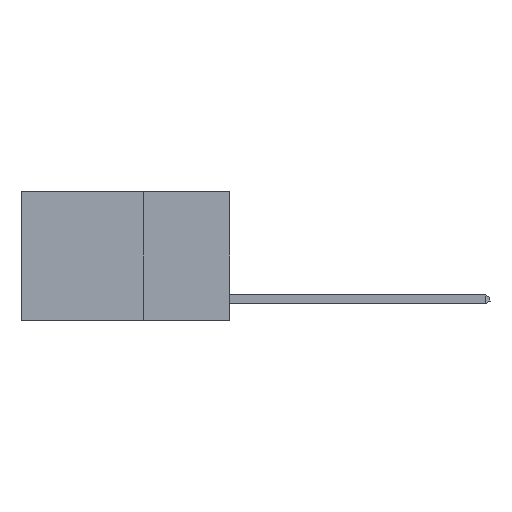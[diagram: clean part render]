
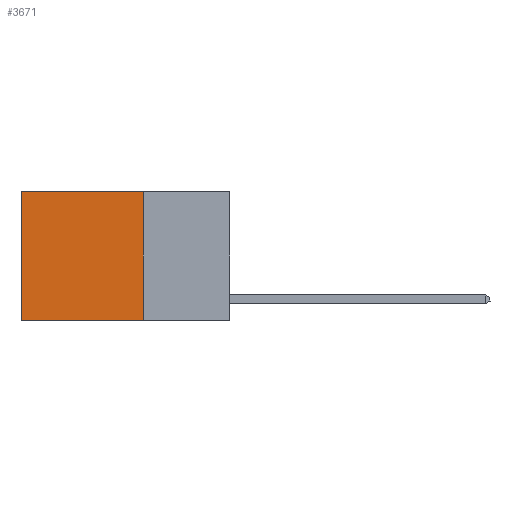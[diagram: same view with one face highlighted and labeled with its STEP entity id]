
A CAD part, left-side view. The second image highlights one B-rep face of the part: STEP entity #3671.
In plain terms, the highlighted planar face has unit normal (-1, 0, 0).
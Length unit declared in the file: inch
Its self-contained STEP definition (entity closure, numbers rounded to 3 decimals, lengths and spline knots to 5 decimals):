
#5 = ORIENTED_EDGE ( 'NONE', *, *, #10603, .F. ) ;
#1289 = CARTESIAN_POINT ( 'NONE',  ( 0.2625, 0.6, 0. ) ) ;
#2048 = CARTESIAN_POINT ( 'NONE',  ( 0.2625, 0.25, 0. ) ) ;
#2095 = CARTESIAN_POINT ( 'NONE',  ( 0.2625, 0.6, 0. ) ) ;
#2175 = VERTEX_POINT ( 'NONE', #13838 ) ;
#2494 = LINE ( 'NONE', #16739, #2633 ) ;
#2633 = VECTOR ( 'NONE', #8717, 39.37008 ) ;
#3352 = EDGE_CURVE ( 'NONE', #10563, #2175, #9768, .T. ) ;
#3671 = ADVANCED_FACE ( 'NONE', ( #4487 ), #16138, .F. ) ;
#3881 = ORIENTED_EDGE ( 'NONE', *, *, #3892, .T. ) ;
#3892 = EDGE_CURVE ( 'NONE', #10563, #13930, #2494, .T. ) ;
#4487 = FACE_OUTER_BOUND ( 'NONE', #5439, .T. ) ;
#4507 = CARTESIAN_POINT ( 'NONE',  ( 0.2625, 0.25, 0. ) ) ;
#5439 = EDGE_LOOP ( 'NONE', ( #5751, #5, #8512, #3881 ) ) ;
#5750 = DIRECTION ( 'NONE',  ( 0., 0., -1. ) ) ;
#5751 = ORIENTED_EDGE ( 'NONE', *, *, #12991, .T. ) ;
#6283 = DIRECTION ( 'NONE',  ( 0., 1., 0. ) ) ;
#6364 = VECTOR ( 'NONE', #15172, 39.37008 ) ;
#8512 = ORIENTED_EDGE ( 'NONE', *, *, #3352, .F. ) ;
#8717 = DIRECTION ( 'NONE',  ( 0., 1., 0. ) ) ;
#9768 = LINE ( 'NONE', #4507, #15367 ) ;
#10563 = VERTEX_POINT ( 'NONE', #13674 ) ;
#10603 = EDGE_CURVE ( 'NONE', #2175, #13217, #12569, .T. ) ;
#10953 = DIRECTION ( 'NONE',  ( 0., 0., -1. ) ) ;
#11899 = VECTOR ( 'NONE', #6283, 39.37008 ) ;
#12327 = CARTESIAN_POINT ( 'NONE',  ( 0.2625, 0.6, -0.37 ) ) ;
#12569 = LINE ( 'NONE', #15158, #11899 ) ;
#12991 = EDGE_CURVE ( 'NONE', #13930, #13217, #14044, .T. ) ;
#13217 = VERTEX_POINT ( 'NONE', #12327 ) ;
#13674 = CARTESIAN_POINT ( 'NONE',  ( 0.2625, 0.25, 0. ) ) ;
#13838 = CARTESIAN_POINT ( 'NONE',  ( 0.2625, 0.25, -0.37 ) ) ;
#13930 = VERTEX_POINT ( 'NONE', #1289 ) ;
#14044 = LINE ( 'NONE', #2095, #6364 ) ;
#14248 = AXIS2_PLACEMENT_3D ( 'NONE', #2048, #14770, #5750 ) ;
#14770 = DIRECTION ( 'NONE',  ( 1., 0., 0. ) ) ;
#15158 = CARTESIAN_POINT ( 'NONE',  ( 0.2625, 0.25, -0.37 ) ) ;
#15172 = DIRECTION ( 'NONE',  ( 0., 0., -1. ) ) ;
#15367 = VECTOR ( 'NONE', #10953, 39.37008 ) ;
#16138 = PLANE ( 'NONE',  #14248 ) ;
#16739 = CARTESIAN_POINT ( 'NONE',  ( 0.2625, 0.25, 0. ) ) ;
